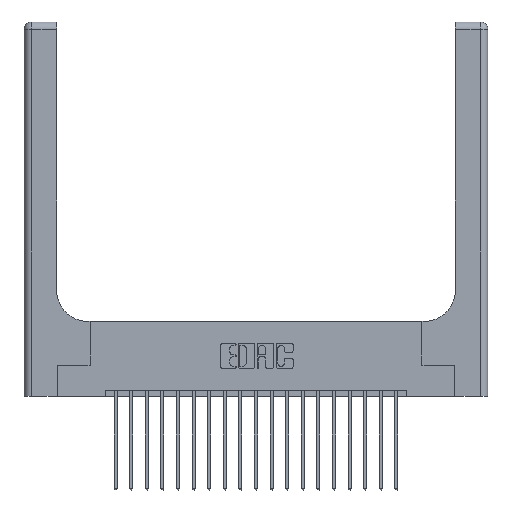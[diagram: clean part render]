
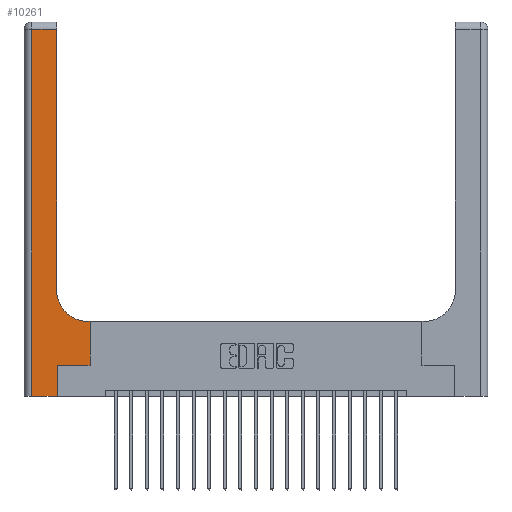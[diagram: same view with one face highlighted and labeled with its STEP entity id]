
A CAD part, top view. The second image highlights one B-rep face of the part: STEP entity #10261.
In plain terms, the highlighted planar face has unit normal (0, 0, 1).
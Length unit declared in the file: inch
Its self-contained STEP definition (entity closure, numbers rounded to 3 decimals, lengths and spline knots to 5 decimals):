
#85 = DIRECTION ( 'NONE',  ( -1., 0., 0. ) ) ;
#310 = CARTESIAN_POINT ( 'NONE',  ( 0.528, 0.6, 0.37 ) ) ;
#540 = VERTEX_POINT ( 'NONE', #10746 ) ;
#987 = CARTESIAN_POINT ( 'NONE',  ( 0.528, 0.25, 0.37 ) ) ;
#988 = LINE ( 'NONE', #9166, #4212 ) ;
#1262 = VECTOR ( 'NONE', #6335, 39.37008 ) ;
#2156 = ORIENTED_EDGE ( 'NONE', *, *, #6400, .T. ) ;
#3042 = CARTESIAN_POINT ( 'NONE',  ( 0.265, 0.25, 0.37 ) ) ;
#3253 = PLANE ( 'NONE',  #11247 ) ;
#3337 = VERTEX_POINT ( 'NONE', #310 ) ;
#3371 = ORIENTED_EDGE ( 'NONE', *, *, #14433, .T. ) ;
#3877 = VECTOR ( 'NONE', #85, 39.37008 ) ;
#4010 = VERTEX_POINT ( 'NONE', #7642 ) ;
#4179 = CARTESIAN_POINT ( 'NONE',  ( 0., 0., 0.37 ) ) ;
#4212 = VECTOR ( 'NONE', #20356, 39.37008 ) ;
#4252 = CARTESIAN_POINT ( 'NONE',  ( 0.265, 0.25, 0.37 ) ) ;
#5153 = CARTESIAN_POINT ( 'NONE',  ( 0.51, 0.6, 0.37 ) ) ;
#6335 = DIRECTION ( 'NONE',  ( 0., 1., 0. ) ) ;
#6370 = ORIENTED_EDGE ( 'NONE', *, *, #16928, .T. ) ;
#6400 = EDGE_CURVE ( 'NONE', #3337, #17457, #10151, .T. ) ;
#7262 = ORIENTED_EDGE ( 'NONE', *, *, #15652, .T. ) ;
#7264 = DIRECTION ( 'NONE',  ( 1., 0., 0. ) ) ;
#7390 = VERTEX_POINT ( 'NONE', #18847 ) ;
#7642 = CARTESIAN_POINT ( 'NONE',  ( 0.26, 0.85, 0.37 ) ) ;
#7751 = DIRECTION ( 'NONE',  ( 1., 0., 0. ) ) ;
#7956 = DIRECTION ( 'NONE',  ( -1., 0., 0. ) ) ;
#8698 = CARTESIAN_POINT ( 'NONE',  ( 0.06, 3., 0.37 ) ) ;
#8850 = AXIS2_PLACEMENT_3D ( 'NONE', #18567, #13448, #7264 ) ;
#8855 = EDGE_CURVE ( 'NONE', #17457, #4010, #19821, .T. ) ;
#8922 = LINE ( 'NONE', #4179, #20669 ) ;
#9003 = ORIENTED_EDGE ( 'NONE', *, *, #10856, .T. ) ;
#9166 = CARTESIAN_POINT ( 'NONE',  ( 0.26, 3., 0.37 ) ) ;
#9477 = CARTESIAN_POINT ( 'NONE',  ( 0.06, 2.94, 0.37 ) ) ;
#9481 = CARTESIAN_POINT ( 'NONE',  ( 0., 3., 0.37 ) ) ;
#9754 = DIRECTION ( 'NONE',  ( 0., 0., -1. ) ) ;
#9795 = ORIENTED_EDGE ( 'NONE', *, *, #16763, .T. ) ;
#9807 = ORIENTED_EDGE ( 'NONE', *, *, #8855, .T. ) ;
#10151 = LINE ( 'NONE', #12604, #3877 ) ;
#10183 = LINE ( 'NONE', #3042, #15174 ) ;
#10243 = ORIENTED_EDGE ( 'NONE', *, *, #10615, .T. ) ;
#10261 = ADVANCED_FACE ( 'NONE', ( #13830 ), #3253, .F. ) ;
#10615 = EDGE_CURVE ( 'NONE', #15083, #19316, #11893, .T. ) ;
#10696 = VERTEX_POINT ( 'NONE', #4252 ) ;
#10746 = CARTESIAN_POINT ( 'NONE',  ( 0.26, 2.94, 0.37 ) ) ;
#10856 = EDGE_CURVE ( 'NONE', #19316, #12624, #8922, .T. ) ;
#10924 = VECTOR ( 'NONE', #11138, 39.37008 ) ;
#11138 = DIRECTION ( 'NONE',  ( 0., 1., 0. ) ) ;
#11247 = AXIS2_PLACEMENT_3D ( 'NONE', #9481, #9754, #7956 ) ;
#11893 = LINE ( 'NONE', #8698, #17677 ) ;
#12604 = CARTESIAN_POINT ( 'NONE',  ( 0.26, 0.6, 0.37 ) ) ;
#12624 = VERTEX_POINT ( 'NONE', #13311 ) ;
#13311 = CARTESIAN_POINT ( 'NONE',  ( 0.265, 0., 0.37 ) ) ;
#13448 = DIRECTION ( 'NONE',  ( 0., 0., -1. ) ) ;
#13731 = DIRECTION ( 'NONE',  ( -1., 0., 0. ) ) ;
#13830 = FACE_OUTER_BOUND ( 'NONE', #18666, .T. ) ;
#14433 = EDGE_CURVE ( 'NONE', #7390, #3337, #17766, .T. ) ;
#15047 = VECTOR ( 'NONE', #13731, 39.37008 ) ;
#15083 = VERTEX_POINT ( 'NONE', #9477 ) ;
#15174 = VECTOR ( 'NONE', #7751, 39.37008 ) ;
#15381 = DIRECTION ( 'NONE',  ( 1., 0., 0. ) ) ;
#15652 = EDGE_CURVE ( 'NONE', #4010, #540, #988, .T. ) ;
#16084 = ORIENTED_EDGE ( 'NONE', *, *, #18818, .T. ) ;
#16763 = EDGE_CURVE ( 'NONE', #10696, #7390, #10183, .T. ) ;
#16928 = EDGE_CURVE ( 'NONE', #12624, #10696, #18425, .T. ) ;
#17457 = VERTEX_POINT ( 'NONE', #5153 ) ;
#17648 = CARTESIAN_POINT ( 'NONE',  ( 0.265, 0., 0.37 ) ) ;
#17677 = VECTOR ( 'NONE', #19877, 39.37008 ) ;
#17766 = LINE ( 'NONE', #987, #1262 ) ;
#18128 = CARTESIAN_POINT ( 'NONE',  ( 0.06, 0., 0.37 ) ) ;
#18425 = LINE ( 'NONE', #17648, #10924 ) ;
#18567 = CARTESIAN_POINT ( 'NONE',  ( 0.51, 0.85, 0.37 ) ) ;
#18630 = CARTESIAN_POINT ( 'NONE',  ( 0., 2.94, 0.37 ) ) ;
#18666 = EDGE_LOOP ( 'NONE', ( #7262, #16084, #10243, #9003, #6370, #9795, #3371, #2156, #9807 ) ) ;
#18818 = EDGE_CURVE ( 'NONE', #540, #15083, #20315, .T. ) ;
#18847 = CARTESIAN_POINT ( 'NONE',  ( 0.528, 0.25, 0.37 ) ) ;
#19316 = VERTEX_POINT ( 'NONE', #18128 ) ;
#19821 = CIRCLE ( 'NONE', #8850, 0.25 ) ;
#19877 = DIRECTION ( 'NONE',  ( 0., -1., 0. ) ) ;
#20315 = LINE ( 'NONE', #18630, #15047 ) ;
#20356 = DIRECTION ( 'NONE',  ( 0., 1., 0. ) ) ;
#20669 = VECTOR ( 'NONE', #15381, 39.37008 ) ;
